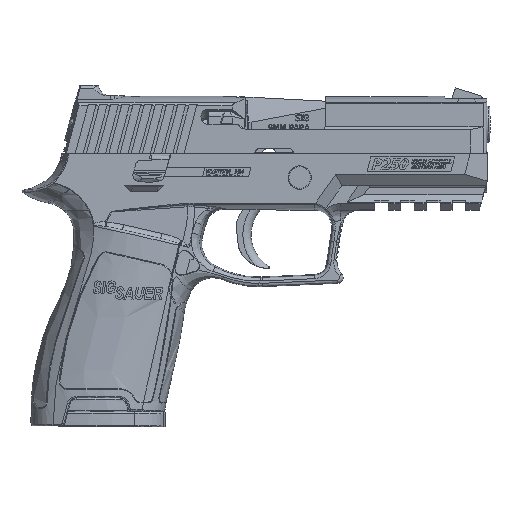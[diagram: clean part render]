
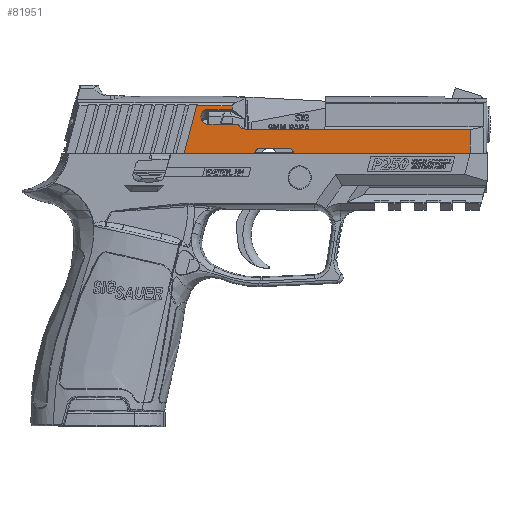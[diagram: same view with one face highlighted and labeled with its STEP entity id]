
A CAD part, top view. The second image highlights one B-rep face of the part: STEP entity #81951.
In plain terms, the highlighted planar face has unit normal (0, 0, 1).
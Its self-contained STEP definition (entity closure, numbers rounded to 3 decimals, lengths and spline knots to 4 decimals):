
#2371=PLANE('',#86776);
#4881=ELLIPSE('',#86780,0.1099,0.09);
#5264=FACE_OUTER_BOUND('',#10008,.T.);
#10008=EDGE_LOOP('',(#56262,#56263,#56264,#56265,#56266,#56267,#56268,#56269,
#56270,#56271,#56272,#56273,#56274,#56275,#56276,#56277));
#15141=CIRCLE('',#86777,0.0745);
#15142=CIRCLE('',#86778,0.0745);
#15143=CIRCLE('',#86779,0.125);
#16807=LINE('',#110976,#24303);
#16826=LINE('',#111149,#24322);
#16829=LINE('',#111155,#24325);
#16830=LINE('',#111157,#24326);
#16831=LINE('',#111161,#24327);
#16832=LINE('',#111165,#24328);
#16833=LINE('',#111167,#24329);
#16834=LINE('',#111169,#24330);
#16835=LINE('',#111171,#24331);
#16836=LINE('',#111173,#24332);
#16837=LINE('',#111177,#24333);
#16838=LINE('',#111180,#24334);
#24303=VECTOR('',#92267,0.5419);
#24322=VECTOR('',#92316,0.0574);
#24325=VECTOR('',#92321,0.7461);
#24326=VECTOR('',#92322,1.0823);
#24327=VECTOR('',#92325,0.439);
#24328=VECTOR('',#92328,2.7012);
#24329=VECTOR('',#92329,0.36);
#24330=VECTOR('',#92330,2.2767);
#24331=VECTOR('',#92331,1.1625);
#24332=VECTOR('',#92332,0.008);
#24333=VECTOR('',#92335,0.4685);
#24334=VECTOR('',#92338,0.386);
#35124=VERTEX_POINT('',#110883);
#35166=VERTEX_POINT('',#110974);
#35197=VERTEX_POINT('',#111148);
#35199=VERTEX_POINT('',#111154);
#35200=VERTEX_POINT('',#111156);
#35201=VERTEX_POINT('',#111158);
#35202=VERTEX_POINT('',#111160);
#35203=VERTEX_POINT('',#111162);
#35204=VERTEX_POINT('',#111164);
#35205=VERTEX_POINT('',#111166);
#35206=VERTEX_POINT('',#111168);
#35207=VERTEX_POINT('',#111170);
#35208=VERTEX_POINT('',#111172);
#35209=VERTEX_POINT('',#111174);
#35210=VERTEX_POINT('',#111176);
#35211=VERTEX_POINT('',#111178);
#43503=EDGE_CURVE('',#35124,#35166,#16807,.T.);
#43539=EDGE_CURVE('',#35197,#35124,#16826,.T.);
#43542=EDGE_CURVE('',#35166,#35199,#16829,.T.);
#43543=EDGE_CURVE('',#35199,#35200,#16830,.T.);
#43544=EDGE_CURVE('',#35200,#35201,#15141,.T.);
#43545=EDGE_CURVE('',#35201,#35202,#16831,.T.);
#43546=EDGE_CURVE('',#35202,#35203,#15142,.T.);
#43547=EDGE_CURVE('',#35203,#35204,#16832,.T.);
#43548=EDGE_CURVE('',#35204,#35205,#16833,.T.);
#43549=EDGE_CURVE('',#35205,#35206,#16834,.T.);
#43550=EDGE_CURVE('',#35206,#35207,#16835,.T.);
#43551=EDGE_CURVE('',#35207,#35208,#16836,.T.);
#43552=EDGE_CURVE('',#35208,#35209,#15143,.T.);
#43553=EDGE_CURVE('',#35209,#35210,#16837,.T.);
#43554=EDGE_CURVE('',#35210,#35211,#4881,.T.);
#43555=EDGE_CURVE('',#35211,#35197,#16838,.T.);
#56262=ORIENTED_EDGE('',*,*,#43503,.T.);
#56263=ORIENTED_EDGE('',*,*,#43542,.T.);
#56264=ORIENTED_EDGE('',*,*,#43543,.T.);
#56265=ORIENTED_EDGE('',*,*,#43544,.T.);
#56266=ORIENTED_EDGE('',*,*,#43545,.T.);
#56267=ORIENTED_EDGE('',*,*,#43546,.T.);
#56268=ORIENTED_EDGE('',*,*,#43547,.T.);
#56269=ORIENTED_EDGE('',*,*,#43548,.T.);
#56270=ORIENTED_EDGE('',*,*,#43549,.T.);
#56271=ORIENTED_EDGE('',*,*,#43550,.T.);
#56272=ORIENTED_EDGE('',*,*,#43551,.T.);
#56273=ORIENTED_EDGE('',*,*,#43552,.T.);
#56274=ORIENTED_EDGE('',*,*,#43553,.T.);
#56275=ORIENTED_EDGE('',*,*,#43554,.T.);
#56276=ORIENTED_EDGE('',*,*,#43555,.T.);
#56277=ORIENTED_EDGE('',*,*,#43539,.T.);
#81951=ADVANCED_FACE('',(#5264),#2371,.T.);
#86776=AXIS2_PLACEMENT_3D('',#111153,#92319,#92320);
#86777=AXIS2_PLACEMENT_3D('',#111159,#92323,#92324);
#86778=AXIS2_PLACEMENT_3D('',#111163,#92326,#92327);
#86779=AXIS2_PLACEMENT_3D('',#111175,#92333,#92334);
#86780=AXIS2_PLACEMENT_3D('',#111179,#92336,#92337);
#92267=DIRECTION('',(-1.,0.,0.));
#92316=DIRECTION('',(0.,1.,0.));
#92319=DIRECTION('center_axis',(0.,0.,1.));
#92320=DIRECTION('ref_axis',(1.,0.,0.));
#92321=DIRECTION('',(-0.259,-0.966,0.));
#92322=DIRECTION('',(1.,0.,0.));
#92323=DIRECTION('center_axis',(0.,0.,-1.));
#92324=DIRECTION('ref_axis',(0.,1.,0.));
#92325=DIRECTION('',(1.,0.,0.));
#92326=DIRECTION('center_axis',(0.,0.,-1.));
#92327=DIRECTION('ref_axis',(1.,0.,0.));
#92328=DIRECTION('',(1.,0.,0.));
#92329=DIRECTION('',(0.,1.,0.));
#92330=DIRECTION('',(-1.,0.,0.));
#92331=DIRECTION('',(-1.,0.,0.));
#92332=DIRECTION('',(0.,1.,0.));
#92333=DIRECTION('center_axis',(0.,0.,-1.));
#92334=DIRECTION('ref_axis',(-0.574,-0.819,0.));
#92335=DIRECTION('',(-1.,0.,0.));
#92336=DIRECTION('center_axis',(0.,0.,-1.));
#92337=DIRECTION('ref_axis',(0.,1.,0.));
#92338=DIRECTION('',(1.,0.,0.));
#110883=CARTESIAN_POINT('',(-0.6322,0.2867,0.5273));
#110974=CARTESIAN_POINT('',(-1.1742,0.2867,0.5273));
#110976=CARTESIAN_POINT('',(-0.405,0.2867,0.5273));
#111148=CARTESIAN_POINT('',(-0.6322,0.2292,0.5273));
#111149=CARTESIAN_POINT('',(-0.6322,0.1812,0.5273));
#111153=CARTESIAN_POINT('Origin',(0.,0.,0.5273));
#111154=CARTESIAN_POINT('',(-1.3673,-0.434,0.5273));
#111155=CARTESIAN_POINT('',(-1.3115,-0.226,0.5273));
#111156=CARTESIAN_POINT('',(-0.285,-0.434,0.5273));
#111157=CARTESIAN_POINT('',(3.253,-0.434,0.5273));
#111158=CARTESIAN_POINT('',(-0.2105,-0.3595,0.5273));
#111159=CARTESIAN_POINT('Origin',(-0.2105,-0.434,
0.5273));
#111160=CARTESIAN_POINT('',(0.2285,-0.3595,0.5273));
#111161=CARTESIAN_POINT('',(-0.1052,-0.3595,0.5273));
#111162=CARTESIAN_POINT('',(0.303,-0.434,0.5273));
#111163=CARTESIAN_POINT('Origin',(0.2285,-0.434,
0.5273));
#111164=CARTESIAN_POINT('',(3.0042,-0.434,0.5273));
#111165=CARTESIAN_POINT('',(3.253,-0.434,0.5273));
#111166=CARTESIAN_POINT('',(3.0042,-0.074,0.5273));
#111167=CARTESIAN_POINT('',(3.0042,-0.217,0.5273));
#111168=CARTESIAN_POINT('',(0.7275,-0.074,0.5273));
#111169=CARTESIAN_POINT('',(-0.2175,-0.074,0.5273));
#111170=CARTESIAN_POINT('',(-0.435,-0.074,0.5273));
#111171=CARTESIAN_POINT('',(-0.2175,-0.074,0.5273));
#111172=CARTESIAN_POINT('',(-0.435,-0.066,0.5273));
#111173=CARTESIAN_POINT('',(-0.435,0.217,0.5273));
#111174=CARTESIAN_POINT('',(-0.5498,0.0095,0.5273));
#111175=CARTESIAN_POINT('Origin',(-0.435,0.059,
0.5273));
#111176=CARTESIAN_POINT('',(-1.0183,0.0095,0.5273));
#111177=CARTESIAN_POINT('',(0.,0.0095,0.5273));
#111178=CARTESIAN_POINT('',(-1.0183,0.2292,0.5273));
#111179=CARTESIAN_POINT('Origin',(-1.0183,0.1194,0.5273));
#111180=CARTESIAN_POINT('',(0.,0.2292,0.5273));
